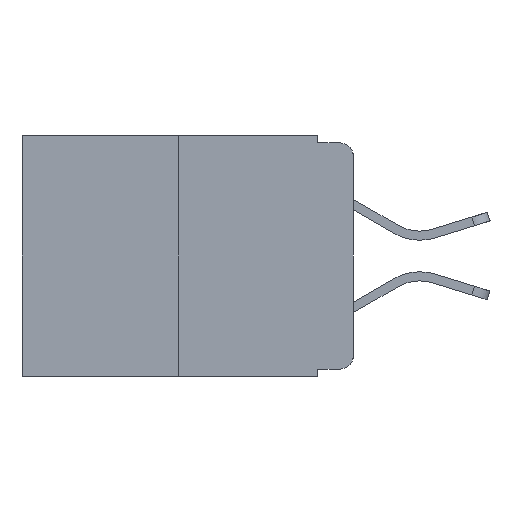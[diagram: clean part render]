
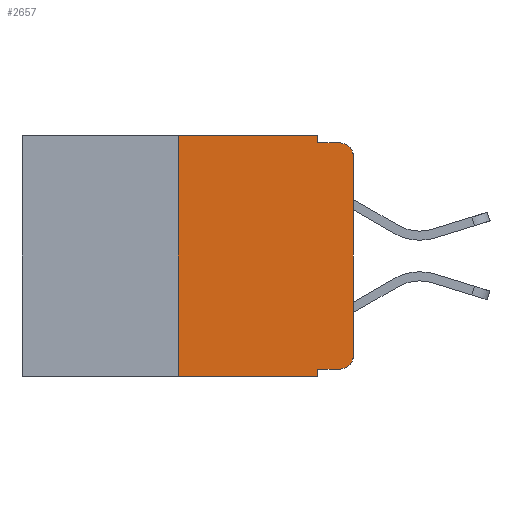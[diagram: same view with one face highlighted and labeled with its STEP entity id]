
A CAD part, left-side view. The second image highlights one B-rep face of the part: STEP entity #2657.
In plain terms, the highlighted planar face has unit normal (-1, 0, 0).
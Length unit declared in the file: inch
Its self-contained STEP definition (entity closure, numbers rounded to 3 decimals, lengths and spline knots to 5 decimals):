
#55 = VECTOR ( 'NONE', #2683, 39.37008 ) ;
#105 = CARTESIAN_POINT ( 'NONE',  ( 0., 0.051, -0.333 ) ) ;
#494 = VERTEX_POINT ( 'NONE', #1808 ) ;
#557 = ORIENTED_EDGE ( 'NONE', *, *, #3557, .F. ) ;
#685 = AXIS2_PLACEMENT_3D ( 'NONE', #8395, #8476, #8499 ) ;
#759 = VERTEX_POINT ( 'NONE', #3377 ) ;
#780 = AXIS2_PLACEMENT_3D ( 'NONE', #7218, #8067, #8049 ) ;
#794 = LINE ( 'NONE', #5918, #2930 ) ;
#940 = EDGE_LOOP ( 'NONE', ( #977, #3400, #4246, #7491, #8913, #557, #3672, #1243, #5010, #7658 ) ) ;
#977 = ORIENTED_EDGE ( 'NONE', *, *, #3398, .T. ) ;
#1243 = ORIENTED_EDGE ( 'NONE', *, *, #3570, .F. ) ;
#1334 = AXIS2_PLACEMENT_3D ( 'NONE', #9113, #7303, #8393 ) ;
#1464 = LINE ( 'NONE', #4862, #7806 ) ;
#1808 = CARTESIAN_POINT ( 'NONE',  ( 0., 0.02, -0.333 ) ) ;
#2078 = LINE ( 'NONE', #4183, #9207 ) ;
#2092 = VECTOR ( 'NONE', #9367, 39.37008 ) ;
#2329 = VERTEX_POINT ( 'NONE', #8939 ) ;
#2509 = LINE ( 'NONE', #7697, #55 ) ;
#2657 = ADVANCED_FACE ( 'NONE', ( #9224 ), #7081, .F. ) ;
#2683 = DIRECTION ( 'NONE',  ( 0., 0., -1. ) ) ;
#2930 = VECTOR ( 'NONE', #6144, 39.37008 ) ;
#3186 = EDGE_CURVE ( 'NONE', #3705, #8624, #8146, .T. ) ;
#3228 = VERTEX_POINT ( 'NONE', #7508 ) ;
#3275 = CARTESIAN_POINT ( 'NONE',  ( 0., 0.25, -0.343 ) ) ;
#3377 = CARTESIAN_POINT ( 'NONE',  ( 0., 0., -0.313 ) ) ;
#3398 = EDGE_CURVE ( 'NONE', #759, #3228, #794, .T. ) ;
#3400 = ORIENTED_EDGE ( 'NONE', *, *, #3415, .T. ) ;
#3415 = EDGE_CURVE ( 'NONE', #3228, #8090, #8464, .T. ) ;
#3469 = EDGE_CURVE ( 'NONE', #6105, #8090, #2078, .T. ) ;
#3484 = EDGE_CURVE ( 'NONE', #5872, #6105, #1464, .T. ) ;
#3557 = EDGE_CURVE ( 'NONE', #3705, #2329, #8534, .T. ) ;
#3570 = EDGE_CURVE ( 'NONE', #5660, #8624, #2509, .T. ) ;
#3575 = EDGE_CURVE ( 'NONE', #5660, #494, #4866, .T. ) ;
#3583 = EDGE_CURVE ( 'NONE', #494, #759, #8223, .T. ) ;
#3672 = ORIENTED_EDGE ( 'NONE', *, *, #3186, .T. ) ;
#3705 = VERTEX_POINT ( 'NONE', #3275 ) ;
#3725 = VECTOR ( 'NONE', #8208, 39.37008 ) ;
#4102 = DIRECTION ( 'NONE',  ( 0., -1., 0. ) ) ;
#4183 = CARTESIAN_POINT ( 'NONE',  ( 0., 0.051, -0.01 ) ) ;
#4246 = ORIENTED_EDGE ( 'NONE', *, *, #3469, .F. ) ;
#4315 = EDGE_CURVE ( 'NONE', #2329, #5872, #9107, .T. ) ;
#4393 = CARTESIAN_POINT ( 'NONE',  ( 0., 0.02, -0.01 ) ) ;
#4593 = VECTOR ( 'NONE', #6548, 39.37008 ) ;
#4862 = CARTESIAN_POINT ( 'NONE',  ( 0., 0.051, 0. ) ) ;
#4866 = LINE ( 'NONE', #6659, #4593 ) ;
#4933 = DIRECTION ( 'NONE',  ( 0., 0., -1. ) ) ;
#5010 = ORIENTED_EDGE ( 'NONE', *, *, #3575, .T. ) ;
#5536 = CARTESIAN_POINT ( 'NONE',  ( 0., 0.051, -0.343 ) ) ;
#5660 = VERTEX_POINT ( 'NONE', #105 ) ;
#5872 = VERTEX_POINT ( 'NONE', #7822 ) ;
#5918 = CARTESIAN_POINT ( 'NONE',  ( 0., 0., 0. ) ) ;
#6105 = VERTEX_POINT ( 'NONE', #7040 ) ;
#6144 = DIRECTION ( 'NONE',  ( 0., 0., 1. ) ) ;
#6548 = DIRECTION ( 'NONE',  ( 0., -1., 0. ) ) ;
#6659 = CARTESIAN_POINT ( 'NONE',  ( 0., 0.051, -0.333 ) ) ;
#6930 = VECTOR ( 'NONE', #7650, 39.37008 ) ;
#7040 = CARTESIAN_POINT ( 'NONE',  ( 0., 0.051, -0.01 ) ) ;
#7081 = PLANE ( 'NONE',  #1334 ) ;
#7218 = CARTESIAN_POINT ( 'NONE',  ( 0., 0.02, -0.03 ) ) ;
#7303 = DIRECTION ( 'NONE',  ( 1., 0., 0. ) ) ;
#7429 = CARTESIAN_POINT ( 'NONE',  ( 0., 0.25, 0. ) ) ;
#7491 = ORIENTED_EDGE ( 'NONE', *, *, #3484, .F. ) ;
#7508 = CARTESIAN_POINT ( 'NONE',  ( 0., 0., -0.03 ) ) ;
#7650 = DIRECTION ( 'NONE',  ( 0., 0., 1. ) ) ;
#7658 = ORIENTED_EDGE ( 'NONE', *, *, #3583, .T. ) ;
#7697 = CARTESIAN_POINT ( 'NONE',  ( 0., 0.051, 0. ) ) ;
#7806 = VECTOR ( 'NONE', #4933, 39.37008 ) ;
#7822 = CARTESIAN_POINT ( 'NONE',  ( 0., 0.051, 0. ) ) ;
#8049 = DIRECTION ( 'NONE',  ( 0., 0., -1. ) ) ;
#8067 = DIRECTION ( 'NONE',  ( -1., 0., 0. ) ) ;
#8090 = VERTEX_POINT ( 'NONE', #4393 ) ;
#8146 = LINE ( 'NONE', #9308, #2092 ) ;
#8208 = DIRECTION ( 'NONE',  ( 0., -1., 0. ) ) ;
#8223 = CIRCLE ( 'NONE', #685, 0.02 ) ;
#8231 = CARTESIAN_POINT ( 'NONE',  ( 0., 0.473, 0. ) ) ;
#8393 = DIRECTION ( 'NONE',  ( 0., 0., -1. ) ) ;
#8395 = CARTESIAN_POINT ( 'NONE',  ( 0., 0.02, -0.313 ) ) ;
#8464 = CIRCLE ( 'NONE', #780, 0.02 ) ;
#8476 = DIRECTION ( 'NONE',  ( -1., 0., 0. ) ) ;
#8499 = DIRECTION ( 'NONE',  ( 0., 0., -1. ) ) ;
#8534 = LINE ( 'NONE', #7429, #6930 ) ;
#8624 = VERTEX_POINT ( 'NONE', #5536 ) ;
#8913 = ORIENTED_EDGE ( 'NONE', *, *, #4315, .F. ) ;
#8939 = CARTESIAN_POINT ( 'NONE',  ( 0., 0.25, 0. ) ) ;
#9107 = LINE ( 'NONE', #8231, #3725 ) ;
#9113 = CARTESIAN_POINT ( 'NONE',  ( 0., 0.473, 0. ) ) ;
#9207 = VECTOR ( 'NONE', #4102, 39.37008 ) ;
#9224 = FACE_OUTER_BOUND ( 'NONE', #940, .T. ) ;
#9308 = CARTESIAN_POINT ( 'NONE',  ( 0., 0.473, -0.343 ) ) ;
#9367 = DIRECTION ( 'NONE',  ( 0., -1., 0. ) ) ;
